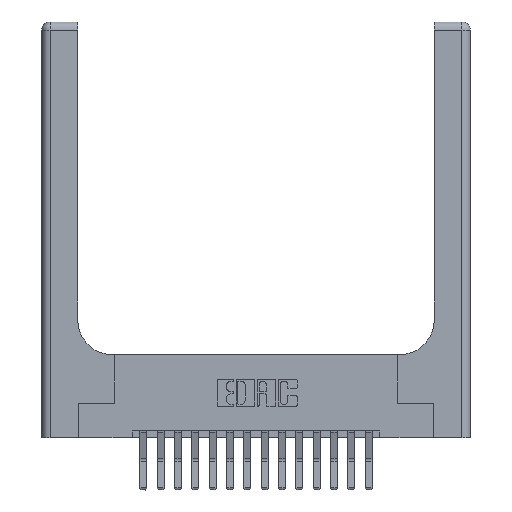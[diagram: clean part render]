
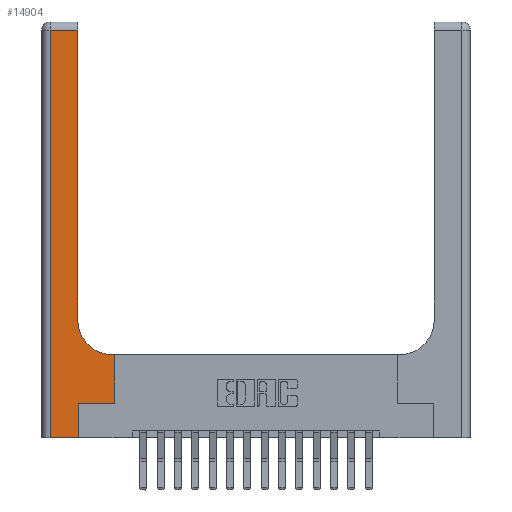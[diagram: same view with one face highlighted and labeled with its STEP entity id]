
A CAD part, top view. The second image highlights one B-rep face of the part: STEP entity #14904.
In plain terms, the highlighted planar face has unit normal (0, 0, 1).
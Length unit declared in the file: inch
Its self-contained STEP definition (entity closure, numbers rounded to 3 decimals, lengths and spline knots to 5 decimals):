
#588 = VERTEX_POINT ( 'NONE', #13569 ) ;
#917 = VERTEX_POINT ( 'NONE', #17053 ) ;
#1159 = CARTESIAN_POINT ( 'NONE',  ( 0.26, 0.6, 0.37 ) ) ;
#1347 = EDGE_CURVE ( 'NONE', #9984, #13226, #15622, .T. ) ;
#1353 = CARTESIAN_POINT ( 'NONE',  ( 0.528, 0.25, 0.37 ) ) ;
#1912 = VERTEX_POINT ( 'NONE', #5652 ) ;
#2227 = CARTESIAN_POINT ( 'NONE',  ( 0., 0., 0.37 ) ) ;
#2252 = EDGE_CURVE ( 'NONE', #3239, #6433, #4365, .T. ) ;
#3239 = VERTEX_POINT ( 'NONE', #17149 ) ;
#3415 = LINE ( 'NONE', #17957, #8717 ) ;
#3730 = DIRECTION ( 'NONE',  ( 1., 0., 0. ) ) ;
#3907 = ORIENTED_EDGE ( 'NONE', *, *, #12673, .T. ) ;
#4365 = CIRCLE ( 'NONE', #13145, 0.25 ) ;
#4751 = EDGE_CURVE ( 'NONE', #1912, #13627, #9579, .T. ) ;
#4864 = EDGE_CURVE ( 'NONE', #917, #9984, #15909, .T. ) ;
#5033 = VERTEX_POINT ( 'NONE', #5990 ) ;
#5652 = CARTESIAN_POINT ( 'NONE',  ( 0.26, 2.94, 0.37 ) ) ;
#5812 = VECTOR ( 'NONE', #15596, 39.37008 ) ;
#5875 = CARTESIAN_POINT ( 'NONE',  ( 0.265, 0.25, 0.37 ) ) ;
#5989 = PLANE ( 'NONE',  #16557 ) ;
#5990 = CARTESIAN_POINT ( 'NONE',  ( 0.06, 0., 0.37 ) ) ;
#6166 = DIRECTION ( 'NONE',  ( 1., 0., 0. ) ) ;
#6184 = DIRECTION ( 'NONE',  ( -1., 0., 0. ) ) ;
#6236 = VECTOR ( 'NONE', #16552, 39.37008 ) ;
#6247 = VECTOR ( 'NONE', #6166, 39.37008 ) ;
#6433 = VERTEX_POINT ( 'NONE', #14417 ) ;
#6479 = EDGE_LOOP ( 'NONE', ( #15074, #8050, #3907, #17709, #8197, #14788, #14448, #6881, #16792 ) ) ;
#6804 = CARTESIAN_POINT ( 'NONE',  ( 0.06, 3., 0.37 ) ) ;
#6881 = ORIENTED_EDGE ( 'NONE', *, *, #15828, .T. ) ;
#7383 = VECTOR ( 'NONE', #16554, 39.37008 ) ;
#8050 = ORIENTED_EDGE ( 'NONE', *, *, #4751, .T. ) ;
#8197 = ORIENTED_EDGE ( 'NONE', *, *, #17503, .T. ) ;
#8378 = CARTESIAN_POINT ( 'NONE',  ( 0., 2.94, 0.37 ) ) ;
#8717 = VECTOR ( 'NONE', #10989, 39.37008 ) ;
#8940 = CARTESIAN_POINT ( 'NONE',  ( 0.06, 2.94, 0.37 ) ) ;
#9378 = DIRECTION ( 'NONE',  ( 1., 0., 0. ) ) ;
#9579 = LINE ( 'NONE', #8378, #5812 ) ;
#9984 = VERTEX_POINT ( 'NONE', #1353 ) ;
#10759 = DIRECTION ( 'NONE',  ( 0., 0., -1. ) ) ;
#10917 = VECTOR ( 'NONE', #12497, 39.37008 ) ;
#10989 = DIRECTION ( 'NONE',  ( 0., 1., 0. ) ) ;
#11078 = DIRECTION ( 'NONE',  ( 0., 1., 0. ) ) ;
#11119 = LINE ( 'NONE', #1159, #10917 ) ;
#11764 = CARTESIAN_POINT ( 'NONE',  ( 0., 3., 0.37 ) ) ;
#11873 = VECTOR ( 'NONE', #11078, 39.37008 ) ;
#12013 = VECTOR ( 'NONE', #9378, 39.37008 ) ;
#12497 = DIRECTION ( 'NONE',  ( -1., 0., 0. ) ) ;
#12673 = EDGE_CURVE ( 'NONE', #13627, #5033, #14202, .T. ) ;
#13145 = AXIS2_PLACEMENT_3D ( 'NONE', #17959, #10759, #3730 ) ;
#13226 = VERTEX_POINT ( 'NONE', #16708 ) ;
#13569 = CARTESIAN_POINT ( 'NONE',  ( 0.265, 0., 0.37 ) ) ;
#13587 = FACE_OUTER_BOUND ( 'NONE', #6479, .T. ) ;
#13627 = VERTEX_POINT ( 'NONE', #8940 ) ;
#13716 = LINE ( 'NONE', #15256, #6236 ) ;
#13911 = CARTESIAN_POINT ( 'NONE',  ( 0.528, 0.25, 0.37 ) ) ;
#14202 = LINE ( 'NONE', #6804, #7383 ) ;
#14417 = CARTESIAN_POINT ( 'NONE',  ( 0.26, 0.85, 0.37 ) ) ;
#14447 = LINE ( 'NONE', #2227, #12013 ) ;
#14448 = ORIENTED_EDGE ( 'NONE', *, *, #1347, .T. ) ;
#14617 = DIRECTION ( 'NONE',  ( 0., 0., -1. ) ) ;
#14788 = ORIENTED_EDGE ( 'NONE', *, *, #4864, .T. ) ;
#14904 = ADVANCED_FACE ( 'NONE', ( #13587 ), #5989, .F. ) ;
#15074 = ORIENTED_EDGE ( 'NONE', *, *, #16434, .T. ) ;
#15256 = CARTESIAN_POINT ( 'NONE',  ( 0.265, 0., 0.37 ) ) ;
#15596 = DIRECTION ( 'NONE',  ( -1., 0., 0. ) ) ;
#15622 = LINE ( 'NONE', #13911, #11873 ) ;
#15805 = EDGE_CURVE ( 'NONE', #5033, #588, #14447, .T. ) ;
#15828 = EDGE_CURVE ( 'NONE', #13226, #3239, #11119, .T. ) ;
#15909 = LINE ( 'NONE', #5875, #6247 ) ;
#16434 = EDGE_CURVE ( 'NONE', #6433, #1912, #3415, .T. ) ;
#16552 = DIRECTION ( 'NONE',  ( 0., 1., 0. ) ) ;
#16554 = DIRECTION ( 'NONE',  ( 0., -1., 0. ) ) ;
#16557 = AXIS2_PLACEMENT_3D ( 'NONE', #11764, #14617, #6184 ) ;
#16708 = CARTESIAN_POINT ( 'NONE',  ( 0.528, 0.6, 0.37 ) ) ;
#16792 = ORIENTED_EDGE ( 'NONE', *, *, #2252, .T. ) ;
#17053 = CARTESIAN_POINT ( 'NONE',  ( 0.265, 0.25, 0.37 ) ) ;
#17149 = CARTESIAN_POINT ( 'NONE',  ( 0.51, 0.6, 0.37 ) ) ;
#17503 = EDGE_CURVE ( 'NONE', #588, #917, #13716, .T. ) ;
#17709 = ORIENTED_EDGE ( 'NONE', *, *, #15805, .T. ) ;
#17957 = CARTESIAN_POINT ( 'NONE',  ( 0.26, 3., 0.37 ) ) ;
#17959 = CARTESIAN_POINT ( 'NONE',  ( 0.51, 0.85, 0.37 ) ) ;
